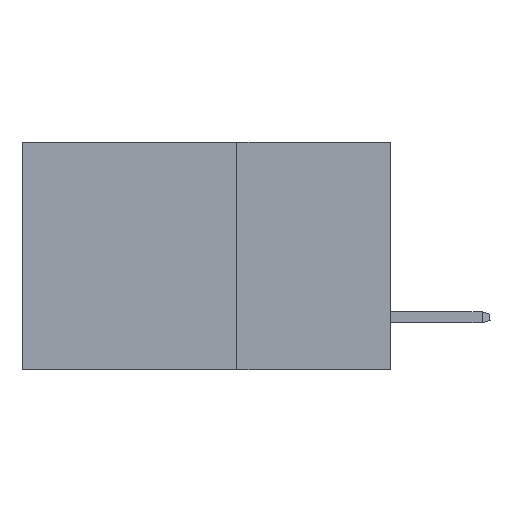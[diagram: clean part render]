
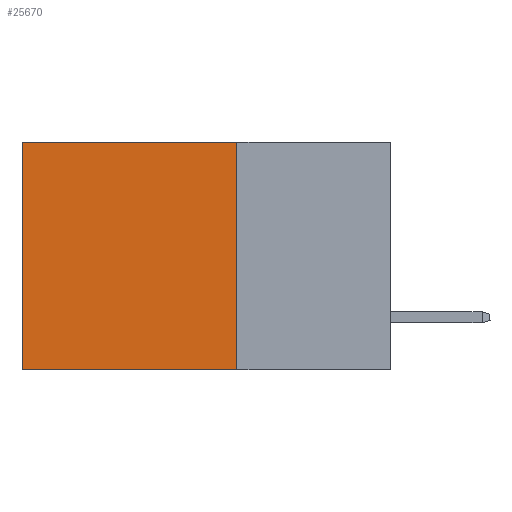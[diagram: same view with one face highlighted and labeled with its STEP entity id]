
A CAD part, left-side view. The second image highlights one B-rep face of the part: STEP entity #25670.
In plain terms, the highlighted planar face has unit normal (-1, 0, 0).
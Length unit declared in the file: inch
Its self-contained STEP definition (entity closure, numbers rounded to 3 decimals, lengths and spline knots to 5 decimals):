
#639 = VECTOR ( 'NONE', #36972, 39.37008 ) ;
#959 = DIRECTION ( 'NONE',  ( 0., 0., -1. ) ) ;
#2071 = CARTESIAN_POINT ( 'NONE',  ( 0.2875, 0.25, 0. ) ) ;
#5374 = VECTOR ( 'NONE', #16856, 39.37008 ) ;
#7226 = LINE ( 'NONE', #40654, #5374 ) ;
#7816 = CARTESIAN_POINT ( 'NONE',  ( 0.2875, 0.6, -0.37 ) ) ;
#8915 = CARTESIAN_POINT ( 'NONE',  ( 0.2875, 0.25, 0. ) ) ;
#9117 = VERTEX_POINT ( 'NONE', #51143 ) ;
#10221 = VECTOR ( 'NONE', #959, 39.37008 ) ;
#11382 = VERTEX_POINT ( 'NONE', #44203 ) ;
#11479 = LINE ( 'NONE', #8915, #10221 ) ;
#13639 = LINE ( 'NONE', #16851, #639 ) ;
#14772 = ORIENTED_EDGE ( 'NONE', *, *, #35751, .T. ) ;
#16327 = ORIENTED_EDGE ( 'NONE', *, *, #18458, .F. ) ;
#16851 = CARTESIAN_POINT ( 'NONE',  ( 0.2875, 0.6, 0. ) ) ;
#16856 = DIRECTION ( 'NONE',  ( 0., 1., 0. ) ) ;
#18458 = EDGE_CURVE ( 'NONE', #9117, #34101, #11479, .T. ) ;
#19009 = FACE_OUTER_BOUND ( 'NONE', #24046, .T. ) ;
#23512 = EDGE_CURVE ( 'NONE', #34101, #30889, #7226, .T. ) ;
#24046 = EDGE_LOOP ( 'NONE', ( #14772, #46623, #16327, #31269 ) ) ;
#24501 = CARTESIAN_POINT ( 'NONE',  ( 0.2875, 0.25, 0. ) ) ;
#25670 = ADVANCED_FACE ( 'NONE', ( #19009 ), #49774, .F. ) ;
#30071 = EDGE_CURVE ( 'NONE', #9117, #11382, #50246, .T. ) ;
#30889 = VERTEX_POINT ( 'NONE', #7816 ) ;
#31269 = ORIENTED_EDGE ( 'NONE', *, *, #30071, .T. ) ;
#34101 = VERTEX_POINT ( 'NONE', #37721 ) ;
#35751 = EDGE_CURVE ( 'NONE', #11382, #30889, #13639, .T. ) ;
#36972 = DIRECTION ( 'NONE',  ( 0., 0., -1. ) ) ;
#37721 = CARTESIAN_POINT ( 'NONE',  ( 0.2875, 0.25, -0.37 ) ) ;
#38119 = DIRECTION ( 'NONE',  ( 0., 0., -1. ) ) ;
#39681 = VECTOR ( 'NONE', #40653, 39.37008 ) ;
#40653 = DIRECTION ( 'NONE',  ( 0., 1., 0. ) ) ;
#40654 = CARTESIAN_POINT ( 'NONE',  ( 0.2875, 0.25, -0.37 ) ) ;
#44203 = CARTESIAN_POINT ( 'NONE',  ( 0.2875, 0.6, 0. ) ) ;
#45608 = DIRECTION ( 'NONE',  ( 1., 0., 0. ) ) ;
#46623 = ORIENTED_EDGE ( 'NONE', *, *, #23512, .F. ) ;
#46648 = AXIS2_PLACEMENT_3D ( 'NONE', #2071, #45608, #38119 ) ;
#49774 = PLANE ( 'NONE',  #46648 ) ;
#50246 = LINE ( 'NONE', #24501, #39681 ) ;
#51143 = CARTESIAN_POINT ( 'NONE',  ( 0.2875, 0.25, 0. ) ) ;
